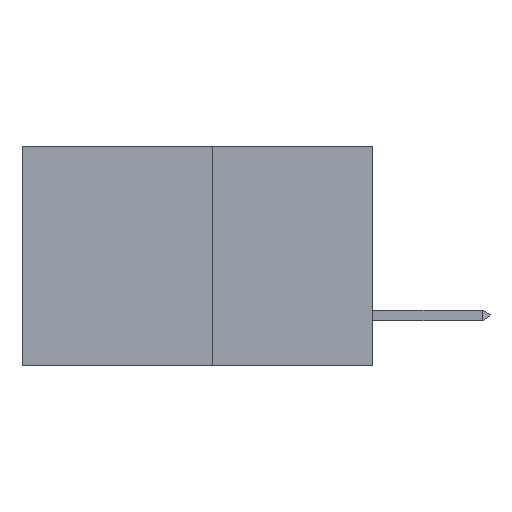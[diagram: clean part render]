
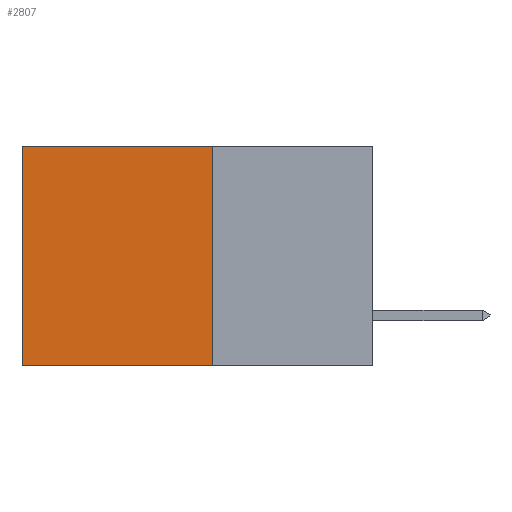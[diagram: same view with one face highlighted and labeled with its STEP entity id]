
A CAD part, left-side view. The second image highlights one B-rep face of the part: STEP entity #2807.
In plain terms, the highlighted planar face has unit normal (-1, 0, 0).
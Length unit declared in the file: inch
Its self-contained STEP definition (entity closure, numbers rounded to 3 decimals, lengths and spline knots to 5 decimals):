
#220 = ORIENTED_EDGE ( 'NONE', *, *, #1009, .F. ) ;
#474 = LINE ( 'NONE', #4809, #6280 ) ;
#692 = ORIENTED_EDGE ( 'NONE', *, *, #6408, .T. ) ;
#777 = ORIENTED_EDGE ( 'NONE', *, *, #8533, .T. ) ;
#1009 = EDGE_CURVE ( 'NONE', #8367, #7913, #474, .T. ) ;
#1036 = VECTOR ( 'NONE', #1746, 39.37008 ) ;
#1289 = ORIENTED_EDGE ( 'NONE', *, *, #9759, .F. ) ;
#1742 = LINE ( 'NONE', #8457, #9571 ) ;
#1746 = DIRECTION ( 'NONE',  ( 0., 1., 0. ) ) ;
#1855 = VECTOR ( 'NONE', #8753, 39.37008 ) ;
#2086 = CARTESIAN_POINT ( 'NONE',  ( 0.277, 0.27, 0. ) ) ;
#2591 = DIRECTION ( 'NONE',  ( 0., 0., -1. ) ) ;
#2807 = ADVANCED_FACE ( 'NONE', ( #9744 ), #6964, .F. ) ;
#3838 = CARTESIAN_POINT ( 'NONE',  ( 0.277, 0.27, -0.37 ) ) ;
#4754 = CARTESIAN_POINT ( 'NONE',  ( 0.277, 0.59, -0.37 ) ) ;
#4809 = CARTESIAN_POINT ( 'NONE',  ( 0.277, 0.27, -0.37 ) ) ;
#5057 = DIRECTION ( 'NONE',  ( 1., 0., 0. ) ) ;
#5557 = LINE ( 'NONE', #7057, #1036 ) ;
#5745 = DIRECTION ( 'NONE',  ( 0., 0., -1. ) ) ;
#5786 = VERTEX_POINT ( 'NONE', #6095 ) ;
#5810 = CARTESIAN_POINT ( 'NONE',  ( 0.277, 0.27, -0.37 ) ) ;
#6095 = CARTESIAN_POINT ( 'NONE',  ( 0.277, 0.59, 0. ) ) ;
#6280 = VECTOR ( 'NONE', #5745, 39.37008 ) ;
#6408 = EDGE_CURVE ( 'NONE', #5786, #8734, #1742, .T. ) ;
#6964 = PLANE ( 'NONE',  #6990 ) ;
#6990 = AXIS2_PLACEMENT_3D ( 'NONE', #5810, #5057, #2591 ) ;
#7057 = CARTESIAN_POINT ( 'NONE',  ( 0.277, 0.27, -0.37 ) ) ;
#7330 = DIRECTION ( 'NONE',  ( 0., 0., -1. ) ) ;
#7913 = VERTEX_POINT ( 'NONE', #3838 ) ;
#8147 = EDGE_LOOP ( 'NONE', ( #692, #1289, #220, #777 ) ) ;
#8367 = VERTEX_POINT ( 'NONE', #8596 ) ;
#8457 = CARTESIAN_POINT ( 'NONE',  ( 0.277, 0.59, -0.37 ) ) ;
#8533 = EDGE_CURVE ( 'NONE', #8367, #5786, #9668, .T. ) ;
#8596 = CARTESIAN_POINT ( 'NONE',  ( 0.277, 0.27, 0. ) ) ;
#8734 = VERTEX_POINT ( 'NONE', #4754 ) ;
#8753 = DIRECTION ( 'NONE',  ( 0., 1., 0. ) ) ;
#9571 = VECTOR ( 'NONE', #7330, 39.37008 ) ;
#9668 = LINE ( 'NONE', #2086, #1855 ) ;
#9744 = FACE_OUTER_BOUND ( 'NONE', #8147, .T. ) ;
#9759 = EDGE_CURVE ( 'NONE', #7913, #8734, #5557, .T. ) ;
